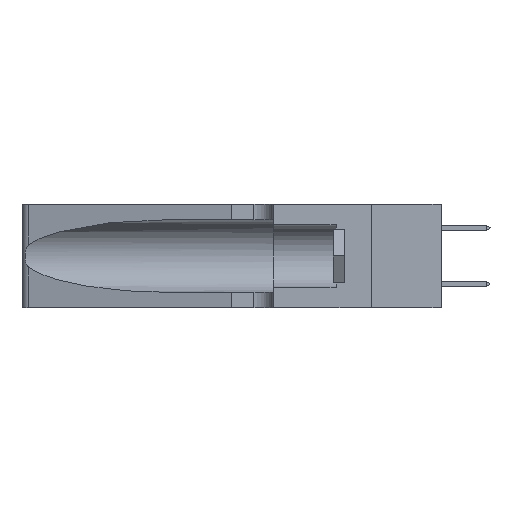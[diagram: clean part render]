
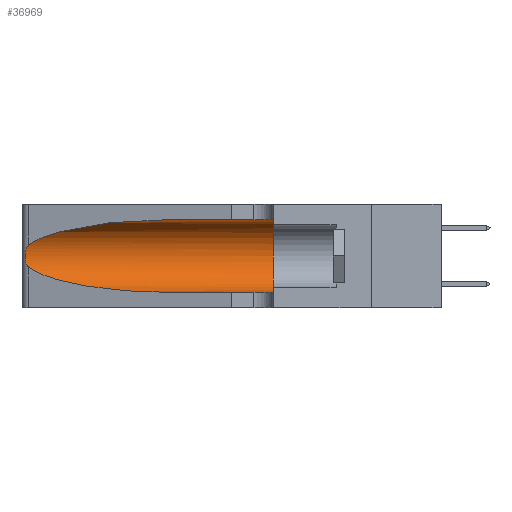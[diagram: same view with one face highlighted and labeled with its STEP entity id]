
A CAD part, left-side view. The second image highlights one B-rep face of the part: STEP entity #36969.
In plain terms, the highlighted cylindrical face has radius 3.308 mm (diameter 6.617 mm), a partial arc.
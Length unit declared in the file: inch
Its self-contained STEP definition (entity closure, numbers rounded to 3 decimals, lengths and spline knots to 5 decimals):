
#1650 = CARTESIAN_POINT ( 'NONE',  ( 0.1305, 0.35, 0.31525 ) ) ;
#1996 = AXIS2_PLACEMENT_3D ( 'NONE', #22601, #4622, #31464 ) ;
#2290 = CARTESIAN_POINT ( 'NONE',  ( 0.25639, 1.23186, 0.15144 ) ) ;
#2374 = VERTEX_POINT ( 'NONE', #1650 ) ;
#2997 = EDGE_CURVE ( 'NONE', #4042, #24521, #22096, .T. ) ;
#3161 = CARTESIAN_POINT ( 'NONE',  ( 0.2373, 1.15595, 0.28018 ) ) ;
#3657 = B_SPLINE_CURVE_WITH_KNOTS ( 'NONE', 3,
 ( #17485, #17230, #29510, #5185, #8208, #14291, #35054, #17354, #38507, #19986, #26050, #2290, #11362, #32543 ),
 .UNSPECIFIED., .F., .F.,
 ( 4, 2, 2, 2, 2, 2, 4 ),
 ( 0., 0.00027, 0.00053, 0.00107, 0.0016, 0.00187, 0.00214 ),
 .UNSPECIFIED. ) ;
#4042 = VERTEX_POINT ( 'NONE', #15175 ) ;
#4622 = DIRECTION ( 'NONE',  ( 0., 1., 0. ) ) ;
#4631 = EDGE_CURVE ( 'NONE', #6029, #4042, #17717, .T. ) ;
#5185 = CARTESIAN_POINT ( 'NONE',  ( 0.25787, 1.23484, 0.2124 ) ) ;
#5492 = DIRECTION ( 'NONE',  ( 0., 0., -1. ) ) ;
#5624 = CARTESIAN_POINT ( 'NONE',  ( 0.1305, 1.61858, 0.185 ) ) ;
#6029 = VERTEX_POINT ( 'NONE', #30917 ) ;
#6488 = EDGE_LOOP ( 'NONE', ( #10363, #19503, #27235, #32446, #20334, #32096 ) ) ;
#7721 = DIRECTION ( 'NONE',  ( 0., -1., 0. ) ) ;
#8208 = CARTESIAN_POINT ( 'NONE',  ( 0.25854, 1.2359, 0.20912 ) ) ;
#9219 = CARTESIAN_POINT ( 'NONE',  ( 0.18966, 0.96281, 0.31525 ) ) ;
#10363 = ORIENTED_EDGE ( 'NONE', *, *, #13494, .T. ) ;
#10437 = FACE_OUTER_BOUND ( 'NONE', #6488, .T. ) ;
#11362 = CARTESIAN_POINT ( 'NONE',  ( 0.25555, 1.22993, 0.14849 ) ) ;
#11363 = CARTESIAN_POINT ( 'NONE',  ( 0.1305, 0.72297, 0.31525 ) ) ;
#13494 = EDGE_CURVE ( 'NONE', #38525, #27240, #15999, .T. ) ;
#13617 = CARTESIAN_POINT ( 'NONE',  ( 0.1305, 0.35, 0.05475 ) ) ;
#14291 = CARTESIAN_POINT ( 'NONE',  ( 0.26018, 1.23835, 0.19895 ) ) ;
#14689 = CYLINDRICAL_SURFACE ( 'NONE', #17585, 0.13025 ) ;
#14739 = CARTESIAN_POINT ( 'NONE',  ( 0.18966, 0.96281, 0.05475 ) ) ;
#14993 = EDGE_CURVE ( 'NONE', #2374, #24521, #28526, .T. ) ;
#15175 = CARTESIAN_POINT ( 'NONE',  ( 0.1305, 0.72297, 0.05475 ) ) ;
#15999 =( BOUNDED_CURVE ( )  B_SPLINE_CURVE ( 3, ( #26914, #9219, #3161, #17958 ),
 .UNSPECIFIED., .F., .F. ) 
 B_SPLINE_CURVE_WITH_KNOTS ( ( 4, 4 ),
 ( 1.5708, 2.84003 ),
 .UNSPECIFIED. ) 
 CURVE ( )  GEOMETRIC_REPRESENTATION_ITEM ( )  RATIONAL_B_SPLINE_CURVE ( ( 1., 0.87, 0.87, 1. ) ) 
 REPRESENTATION_ITEM ( '' )  );
#17230 = CARTESIAN_POINT ( 'NONE',  ( 0.25555, 1.22994, 0.2215 ) ) ;
#17354 = CARTESIAN_POINT ( 'NONE',  ( 0.26075, 1.23896, 0.178 ) ) ;
#17485 = CARTESIAN_POINT ( 'NONE',  ( 0.25487, 1.22718, 0.22369 ) ) ;
#17585 = AXIS2_PLACEMENT_3D ( 'NONE', #5624, #35224, #5492 ) ;
#17717 =( BOUNDED_CURVE ( )  B_SPLINE_CURVE ( 3, ( #24257, #30094, #14739, #26882 ),
 .UNSPECIFIED., .F., .F. ) 
 B_SPLINE_CURVE_WITH_KNOTS ( ( 4, 4 ),
 ( 3.44316, 4.71239 ),
 .UNSPECIFIED. ) 
 CURVE ( )  GEOMETRIC_REPRESENTATION_ITEM ( )  RATIONAL_B_SPLINE_CURVE ( ( 1., 0.87, 0.87, 1. ) ) 
 REPRESENTATION_ITEM ( '' )  );
#17958 = CARTESIAN_POINT ( 'NONE',  ( 0.25487, 1.22718, 0.22369 ) ) ;
#17970 = EDGE_CURVE ( 'NONE', #27240, #6029, #3657, .T. ) ;
#18207 = LINE ( 'NONE', #26081, #23383 ) ;
#19109 = EDGE_CURVE ( 'NONE', #38525, #2374, #18207, .T. ) ;
#19503 = ORIENTED_EDGE ( 'NONE', *, *, #17970, .T. ) ;
#19986 = CARTESIAN_POINT ( 'NONE',  ( 0.25856, 1.23593, 0.16098 ) ) ;
#20334 = ORIENTED_EDGE ( 'NONE', *, *, #14993, .F. ) ;
#21797 = CARTESIAN_POINT ( 'NONE',  ( 0.1305, 1.61858, 0.05475 ) ) ;
#22096 = LINE ( 'NONE', #21797, #24007 ) ;
#22601 = CARTESIAN_POINT ( 'NONE',  ( 0.1305, 0.35, 0.185 ) ) ;
#23383 = VECTOR ( 'NONE', #7721, 39.37008 ) ;
#24007 = VECTOR ( 'NONE', #30936, 39.37008 ) ;
#24257 = CARTESIAN_POINT ( 'NONE',  ( 0.25487, 1.22718, 0.14631 ) ) ;
#24521 = VERTEX_POINT ( 'NONE', #13617 ) ;
#25210 = CARTESIAN_POINT ( 'NONE',  ( 0.25487, 1.22718, 0.22369 ) ) ;
#26050 = CARTESIAN_POINT ( 'NONE',  ( 0.25789, 1.23486, 0.15765 ) ) ;
#26081 = CARTESIAN_POINT ( 'NONE',  ( 0.1305, 1.61858, 0.31525 ) ) ;
#26882 = CARTESIAN_POINT ( 'NONE',  ( 0.1305, 0.72297, 0.05475 ) ) ;
#26914 = CARTESIAN_POINT ( 'NONE',  ( 0.1305, 0.72297, 0.31525 ) ) ;
#27235 = ORIENTED_EDGE ( 'NONE', *, *, #4631, .T. ) ;
#27240 = VERTEX_POINT ( 'NONE', #25210 ) ;
#28526 = CIRCLE ( 'NONE', #1996, 0.13025 ) ;
#29510 = CARTESIAN_POINT ( 'NONE',  ( 0.25639, 1.23184, 0.21858 ) ) ;
#30094 = CARTESIAN_POINT ( 'NONE',  ( 0.2373, 1.15595, 0.08982 ) ) ;
#30917 = CARTESIAN_POINT ( 'NONE',  ( 0.25487, 1.22718, 0.14631 ) ) ;
#30936 = DIRECTION ( 'NONE',  ( 0., -1., 0. ) ) ;
#31464 = DIRECTION ( 'NONE',  ( 0., 0., 1. ) ) ;
#32096 = ORIENTED_EDGE ( 'NONE', *, *, #19109, .F. ) ;
#32446 = ORIENTED_EDGE ( 'NONE', *, *, #2997, .T. ) ;
#32543 = CARTESIAN_POINT ( 'NONE',  ( 0.25487, 1.22718, 0.14631 ) ) ;
#35054 = CARTESIAN_POINT ( 'NONE',  ( 0.26075, 1.23896, 0.19203 ) ) ;
#35224 = DIRECTION ( 'NONE',  ( 0., -1., 0. ) ) ;
#36969 = ADVANCED_FACE ( 'NONE', ( #10437 ), #14689, .F. ) ;
#38507 = CARTESIAN_POINT ( 'NONE',  ( 0.26017, 1.23833, 0.17102 ) ) ;
#38525 = VERTEX_POINT ( 'NONE', #11363 ) ;
